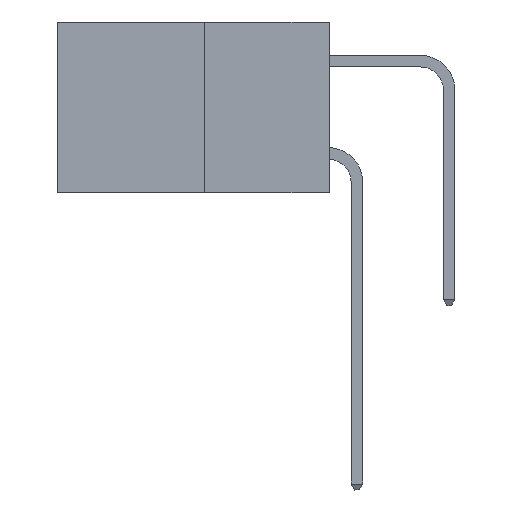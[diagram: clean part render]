
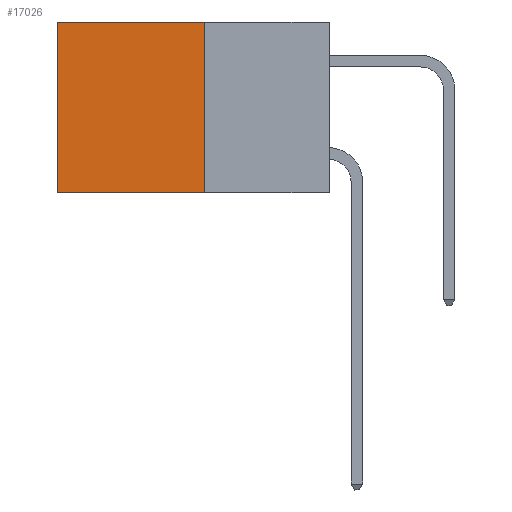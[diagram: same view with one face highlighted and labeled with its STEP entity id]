
A CAD part, left-side view. The second image highlights one B-rep face of the part: STEP entity #17026.
In plain terms, the highlighted planar face has unit normal (-1, 0, 0).
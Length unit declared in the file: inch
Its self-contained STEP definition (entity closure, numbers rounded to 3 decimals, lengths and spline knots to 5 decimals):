
#1644 = DIRECTION ( 'NONE',  ( 0., 0., -1. ) ) ;
#2098 = VECTOR ( 'NONE', #1644, 39.37008 ) ;
#2956 = DIRECTION ( 'NONE',  ( 0., 0., -1. ) ) ;
#3611 = EDGE_CURVE ( 'NONE', #8643, #5484, #4773, .T. ) ;
#3777 = ORIENTED_EDGE ( 'NONE', *, *, #20628, .F. ) ;
#4773 = LINE ( 'NONE', #9238, #19368 ) ;
#4878 = CARTESIAN_POINT ( 'NONE',  ( 0.277, 0.27, 0. ) ) ;
#4904 = AXIS2_PLACEMENT_3D ( 'NONE', #7802, #21583, #9836 ) ;
#5484 = VERTEX_POINT ( 'NONE', #20593 ) ;
#5660 = LINE ( 'NONE', #16246, #16265 ) ;
#6326 = DIRECTION ( 'NONE',  ( 0., 1., 0. ) ) ;
#6946 = DIRECTION ( 'NONE',  ( 0., 1., 0. ) ) ;
#7364 = VERTEX_POINT ( 'NONE', #21231 ) ;
#7473 = LINE ( 'NONE', #19558, #2098 ) ;
#7802 = CARTESIAN_POINT ( 'NONE',  ( 0.277, 0.27, -0.37 ) ) ;
#8643 = VERTEX_POINT ( 'NONE', #22262 ) ;
#8824 = ORIENTED_EDGE ( 'NONE', *, *, #18927, .F. ) ;
#9238 = CARTESIAN_POINT ( 'NONE',  ( 0.277, 0.59, -0.37 ) ) ;
#9836 = DIRECTION ( 'NONE',  ( 0., 0., -1. ) ) ;
#10019 = VERTEX_POINT ( 'NONE', #14942 ) ;
#10414 = LINE ( 'NONE', #4878, #25332 ) ;
#13529 = EDGE_LOOP ( 'NONE', ( #17473, #8824, #3777, #14477 ) ) ;
#14247 = FACE_OUTER_BOUND ( 'NONE', #13529, .T. ) ;
#14477 = ORIENTED_EDGE ( 'NONE', *, *, #22243, .T. ) ;
#14942 = CARTESIAN_POINT ( 'NONE',  ( 0.277, 0.27, 0. ) ) ;
#16246 = CARTESIAN_POINT ( 'NONE',  ( 0.277, 0.27, -0.37 ) ) ;
#16265 = VECTOR ( 'NONE', #6326, 39.37008 ) ;
#17026 = ADVANCED_FACE ( 'NONE', ( #14247 ), #19609, .F. ) ;
#17473 = ORIENTED_EDGE ( 'NONE', *, *, #3611, .T. ) ;
#18927 = EDGE_CURVE ( 'NONE', #7364, #5484, #5660, .T. ) ;
#19368 = VECTOR ( 'NONE', #2956, 39.37008 ) ;
#19558 = CARTESIAN_POINT ( 'NONE',  ( 0.277, 0.27, -0.37 ) ) ;
#19609 = PLANE ( 'NONE',  #4904 ) ;
#20593 = CARTESIAN_POINT ( 'NONE',  ( 0.277, 0.59, -0.37 ) ) ;
#20628 = EDGE_CURVE ( 'NONE', #10019, #7364, #7473, .T. ) ;
#21231 = CARTESIAN_POINT ( 'NONE',  ( 0.277, 0.27, -0.37 ) ) ;
#21583 = DIRECTION ( 'NONE',  ( 1., 0., 0. ) ) ;
#22243 = EDGE_CURVE ( 'NONE', #10019, #8643, #10414, .T. ) ;
#22262 = CARTESIAN_POINT ( 'NONE',  ( 0.277, 0.59, 0. ) ) ;
#25332 = VECTOR ( 'NONE', #6946, 39.37008 ) ;
